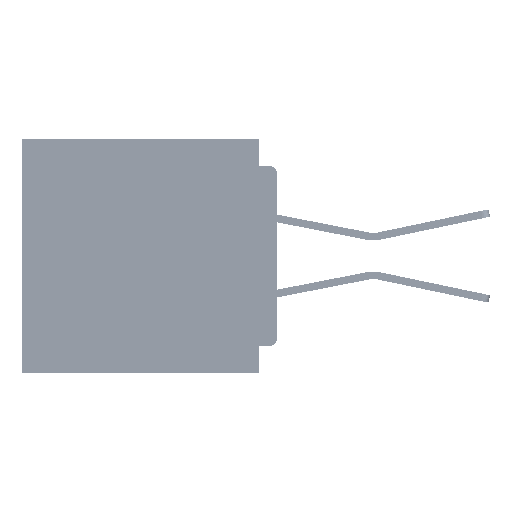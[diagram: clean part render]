
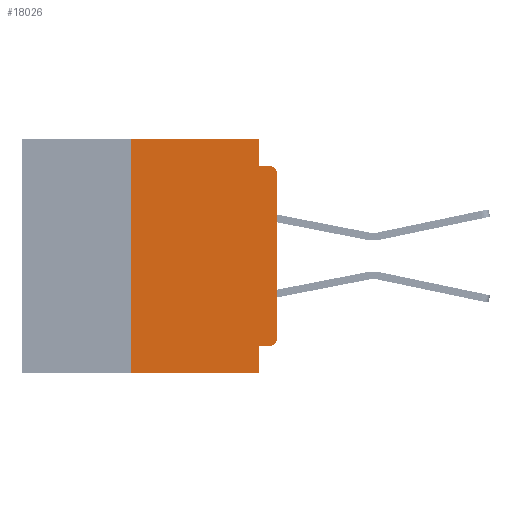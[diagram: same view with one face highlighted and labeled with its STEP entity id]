
A CAD part, left-side view. The second image highlights one B-rep face of the part: STEP entity #18026.
In plain terms, the highlighted planar face has unit normal (-1, 0, 0).
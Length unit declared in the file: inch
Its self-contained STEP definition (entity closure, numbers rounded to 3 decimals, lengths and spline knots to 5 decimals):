
#939 = LINE ( 'NONE', #66385, #55609 ) ;
#1149 = CARTESIAN_POINT ( 'NONE',  ( 0., 0.015, -0.045 ) ) ;
#2441 = PLANE ( 'NONE',  #18935 ) ;
#3028 = EDGE_CURVE ( 'NONE', #36031, #53652, #8545, .T. ) ;
#4600 = CARTESIAN_POINT ( 'NONE',  ( 0., 0., -0.355 ) ) ;
#6378 = DIRECTION ( 'NONE',  ( 0., 0., -1. ) ) ;
#6497 = CIRCLE ( 'NONE', #28176, 0.015 ) ;
#6858 = CARTESIAN_POINT ( 'NONE',  ( 0., 0.031, 0. ) ) ;
#7210 = CARTESIAN_POINT ( 'NONE',  ( 0., 0.25, -0.4 ) ) ;
#8545 = LINE ( 'NONE', #6858, #63138 ) ;
#9065 = VECTOR ( 'NONE', #51563, 39.37008 ) ;
#10874 = FACE_OUTER_BOUND ( 'NONE', #25733, .T. ) ;
#11151 = EDGE_CURVE ( 'NONE', #35605, #56090, #6497, .T. ) ;
#11256 = VECTOR ( 'NONE', #20816, 39.37008 ) ;
#11356 = EDGE_CURVE ( 'NONE', #20112, #36031, #21830, .T. ) ;
#11494 = CARTESIAN_POINT ( 'NONE',  ( 0., 0.015, -0.06 ) ) ;
#11807 = CARTESIAN_POINT ( 'NONE',  ( 0., 0.015, -0.34 ) ) ;
#12965 = LINE ( 'NONE', #4600, #11256 ) ;
#13439 = VERTEX_POINT ( 'NONE', #7210 ) ;
#13452 = CARTESIAN_POINT ( 'NONE',  ( 0., 0.437, 0. ) ) ;
#13473 = CARTESIAN_POINT ( 'NONE',  ( 0., 0.437, 0. ) ) ;
#16223 = CARTESIAN_POINT ( 'NONE',  ( 0., 0., -0.34 ) ) ;
#16947 = DIRECTION ( 'NONE',  ( 0., 0., -1. ) ) ;
#17273 = DIRECTION ( 'NONE',  ( 0., 0., -1. ) ) ;
#17347 = ORIENTED_EDGE ( 'NONE', *, *, #40076, .F. ) ;
#17415 = VECTOR ( 'NONE', #56016, 39.37008 ) ;
#18026 = ADVANCED_FACE ( 'NONE', ( #10874 ), #2441, .F. ) ;
#18935 = AXIS2_PLACEMENT_3D ( 'NONE', #13473, #62566, #29853 ) ;
#18995 = LINE ( 'NONE', #38603, #47983 ) ;
#20112 = VERTEX_POINT ( 'NONE', #31014 ) ;
#20816 = DIRECTION ( 'NONE',  ( 0., 1., 0. ) ) ;
#21233 = ORIENTED_EDGE ( 'NONE', *, *, #70571, .F. ) ;
#21830 = LINE ( 'NONE', #13452, #9065 ) ;
#21860 = DIRECTION ( 'NONE',  ( 0., -1., 0. ) ) ;
#23291 = ORIENTED_EDGE ( 'NONE', *, *, #57302, .F. ) ;
#24257 = CARTESIAN_POINT ( 'NONE',  ( 0., 0.031, -0.4 ) ) ;
#24396 = EDGE_CURVE ( 'NONE', #61004, #61260, #55597, .T. ) ;
#24675 = CARTESIAN_POINT ( 'NONE',  ( 0., 0.031, 0. ) ) ;
#25733 = EDGE_LOOP ( 'NONE', ( #39784, #56352, #21233, #42800, #48148, #39540, #37341, #17347, #23291, #62533 ) ) ;
#26490 = CARTESIAN_POINT ( 'NONE',  ( 0., 0., -0.06 ) ) ;
#28176 = AXIS2_PLACEMENT_3D ( 'NONE', #11807, #49908, #17273 ) ;
#29853 = DIRECTION ( 'NONE',  ( 0., 0., -1. ) ) ;
#31014 = CARTESIAN_POINT ( 'NONE',  ( 0., 0.25, 0. ) ) ;
#31872 = LINE ( 'NONE', #39577, #17415 ) ;
#32815 = CARTESIAN_POINT ( 'NONE',  ( 0., 0., -0.045 ) ) ;
#34296 = EDGE_CURVE ( 'NONE', #56090, #61004, #939, .T. ) ;
#35605 = VERTEX_POINT ( 'NONE', #58340 ) ;
#36031 = VERTEX_POINT ( 'NONE', #24675 ) ;
#37341 = ORIENTED_EDGE ( 'NONE', *, *, #44638, .T. ) ;
#38364 = DIRECTION ( 'NONE',  ( 0., 0., -1. ) ) ;
#38603 = CARTESIAN_POINT ( 'NONE',  ( 0., 0.031, -0.4 ) ) ;
#39540 = ORIENTED_EDGE ( 'NONE', *, *, #70232, .F. ) ;
#39577 = CARTESIAN_POINT ( 'NONE',  ( 0., 0.25, -0.4 ) ) ;
#39784 = ORIENTED_EDGE ( 'NONE', *, *, #34296, .T. ) ;
#40076 = EDGE_CURVE ( 'NONE', #43407, #49826, #18995, .T. ) ;
#42800 = ORIENTED_EDGE ( 'NONE', *, *, #3028, .F. ) ;
#43407 = VERTEX_POINT ( 'NONE', #70397 ) ;
#44638 = EDGE_CURVE ( 'NONE', #13439, #49826, #60192, .T. ) ;
#45678 = VECTOR ( 'NONE', #65503, 39.37008 ) ;
#46327 = CARTESIAN_POINT ( 'NONE',  ( 0., 0.031, -0.045 ) ) ;
#47983 = VECTOR ( 'NONE', #38364, 39.37008 ) ;
#48148 = ORIENTED_EDGE ( 'NONE', *, *, #11356, .F. ) ;
#48801 = AXIS2_PLACEMENT_3D ( 'NONE', #11494, #49586, #16947 ) ;
#49586 = DIRECTION ( 'NONE',  ( -1., 0., 0. ) ) ;
#49826 = VERTEX_POINT ( 'NONE', #24257 ) ;
#49908 = DIRECTION ( 'NONE',  ( -1., 0., 0. ) ) ;
#50083 = DIRECTION ( 'NONE',  ( 0., 0., 1. ) ) ;
#51563 = DIRECTION ( 'NONE',  ( 0., -1., 0. ) ) ;
#53652 = VERTEX_POINT ( 'NONE', #46327 ) ;
#54520 = CARTESIAN_POINT ( 'NONE',  ( 0., 0.437, -0.4 ) ) ;
#55597 = CIRCLE ( 'NONE', #48801, 0.015 ) ;
#55609 = VECTOR ( 'NONE', #50083, 39.37008 ) ;
#56016 = DIRECTION ( 'NONE',  ( 0., 0., 1. ) ) ;
#56090 = VERTEX_POINT ( 'NONE', #16223 ) ;
#56352 = ORIENTED_EDGE ( 'NONE', *, *, #24396, .T. ) ;
#57302 = EDGE_CURVE ( 'NONE', #35605, #43407, #12965, .T. ) ;
#58340 = CARTESIAN_POINT ( 'NONE',  ( 0., 0.015, -0.355 ) ) ;
#60192 = LINE ( 'NONE', #54520, #45678 ) ;
#61004 = VERTEX_POINT ( 'NONE', #26490 ) ;
#61260 = VERTEX_POINT ( 'NONE', #1149 ) ;
#62533 = ORIENTED_EDGE ( 'NONE', *, *, #11151, .T. ) ;
#62566 = DIRECTION ( 'NONE',  ( 1., 0., 0. ) ) ;
#63138 = VECTOR ( 'NONE', #6378, 39.37008 ) ;
#64285 = VECTOR ( 'NONE', #21860, 39.37008 ) ;
#65503 = DIRECTION ( 'NONE',  ( 0., -1., 0. ) ) ;
#66015 = LINE ( 'NONE', #32815, #64285 ) ;
#66385 = CARTESIAN_POINT ( 'NONE',  ( 0., 0., 0. ) ) ;
#70232 = EDGE_CURVE ( 'NONE', #13439, #20112, #31872, .T. ) ;
#70397 = CARTESIAN_POINT ( 'NONE',  ( 0., 0.031, -0.355 ) ) ;
#70571 = EDGE_CURVE ( 'NONE', #53652, #61260, #66015, .T. ) ;
